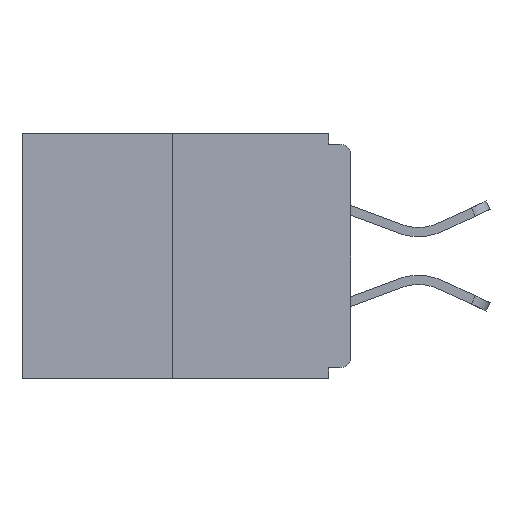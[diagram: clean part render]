
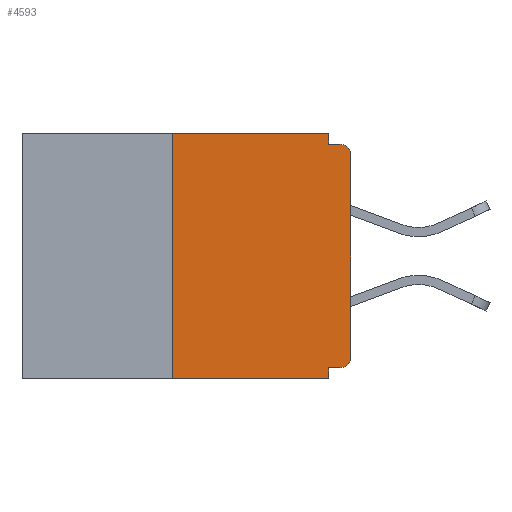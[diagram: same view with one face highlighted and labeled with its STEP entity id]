
A CAD part, left-side view. The second image highlights one B-rep face of the part: STEP entity #4593.
In plain terms, the highlighted planar face has unit normal (-1, 0, 0).
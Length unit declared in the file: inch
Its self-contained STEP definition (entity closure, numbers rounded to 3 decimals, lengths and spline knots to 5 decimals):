
#441 = LINE ( 'NONE', #9095, #3530 ) ;
#461 = VERTEX_POINT ( 'NONE', #24183 ) ;
#647 = DIRECTION ( 'NONE',  ( 0., -1., 0. ) ) ;
#723 = CARTESIAN_POINT ( 'NONE',  ( 0., 0.25, -0.343 ) ) ;
#873 = ORIENTED_EDGE ( 'NONE', *, *, #22723, .T. ) ;
#1362 = AXIS2_PLACEMENT_3D ( 'NONE', #7257, #23128, #17271 ) ;
#1671 = CARTESIAN_POINT ( 'NONE',  ( 0., 0.25, 0. ) ) ;
#1833 = CIRCLE ( 'NONE', #21956, 0.015 ) ;
#2338 = CARTESIAN_POINT ( 'NONE',  ( 0., 0.46, 0. ) ) ;
#2675 = EDGE_CURVE ( 'NONE', #16763, #24442, #19767, .T. ) ;
#3530 = VECTOR ( 'NONE', #11097, 39.37008 ) ;
#3988 = DIRECTION ( 'NONE',  ( 0., 0., 1. ) ) ;
#4593 = ADVANCED_FACE ( 'NONE', ( #5600 ), #15111, .F. ) ;
#4710 = DIRECTION ( 'NONE',  ( -1., 0., 0. ) ) ;
#4755 = VECTOR ( 'NONE', #13720, 39.37008 ) ;
#5445 = DIRECTION ( 'NONE',  ( 0., 0., -1. ) ) ;
#5600 = FACE_OUTER_BOUND ( 'NONE', #6929, .T. ) ;
#5951 = CARTESIAN_POINT ( 'NONE',  ( 0., 0., -0.015 ) ) ;
#6776 = CARTESIAN_POINT ( 'NONE',  ( 0., 0.031, -0.343 ) ) ;
#6848 = CARTESIAN_POINT ( 'NONE',  ( 0., 0.031, -0.343 ) ) ;
#6924 = CARTESIAN_POINT ( 'NONE',  ( 0., 0.031, 0. ) ) ;
#6929 = EDGE_LOOP ( 'NONE', ( #24272, #15865, #21165, #22996, #10280, #16289, #873, #14634, #24506, #10809 ) ) ;
#7257 = CARTESIAN_POINT ( 'NONE',  ( 0., 0.46, 0. ) ) ;
#7314 = CARTESIAN_POINT ( 'NONE',  ( 0., 0.015, -0.015 ) ) ;
#7361 = CARTESIAN_POINT ( 'NONE',  ( 0., 0.031, 0. ) ) ;
#7460 = LINE ( 'NONE', #6848, #10587 ) ;
#8065 = DIRECTION ( 'NONE',  ( 0., 0., -1. ) ) ;
#8109 = CARTESIAN_POINT ( 'NONE',  ( 0., 0., 0. ) ) ;
#8378 = DIRECTION ( 'NONE',  ( 0., -1., 0. ) ) ;
#8689 = VERTEX_POINT ( 'NONE', #7361 ) ;
#9004 = VECTOR ( 'NONE', #647, 39.37008 ) ;
#9095 = CARTESIAN_POINT ( 'NONE',  ( 0., 0.25, 0. ) ) ;
#9222 = EDGE_CURVE ( 'NONE', #15739, #12698, #18220, .T. ) ;
#9432 = VERTEX_POINT ( 'NONE', #9999 ) ;
#9542 = CARTESIAN_POINT ( 'NONE',  ( 0., 0.031, -0.328 ) ) ;
#9869 = CARTESIAN_POINT ( 'NONE',  ( 0., 0.031, -0.015 ) ) ;
#9999 = CARTESIAN_POINT ( 'NONE',  ( 0., 0., -0.03 ) ) ;
#10280 = ORIENTED_EDGE ( 'NONE', *, *, #9222, .F. ) ;
#10587 = VECTOR ( 'NONE', #5445, 39.37008 ) ;
#10809 = ORIENTED_EDGE ( 'NONE', *, *, #21538, .F. ) ;
#11043 = LINE ( 'NONE', #2338, #20100 ) ;
#11097 = DIRECTION ( 'NONE',  ( 0., 0., 1. ) ) ;
#11209 = VERTEX_POINT ( 'NONE', #1671 ) ;
#11656 = DIRECTION ( 'NONE',  ( 0., 1., 0. ) ) ;
#11887 = DIRECTION ( 'NONE',  ( -1., 0., 0. ) ) ;
#12581 = EDGE_CURVE ( 'NONE', #12698, #21178, #7460, .T. ) ;
#12598 = DIRECTION ( 'NONE',  ( 0., 0., -1. ) ) ;
#12698 = VERTEX_POINT ( 'NONE', #9542 ) ;
#12739 = EDGE_CURVE ( 'NONE', #15739, #461, #19937, .T. ) ;
#12963 = EDGE_CURVE ( 'NONE', #20572, #21178, #23593, .T. ) ;
#13240 = AXIS2_PLACEMENT_3D ( 'NONE', #15998, #11887, #8065 ) ;
#13720 = DIRECTION ( 'NONE',  ( 0., -1., 0. ) ) ;
#14511 = VECTOR ( 'NONE', #12598, 39.37008 ) ;
#14634 = ORIENTED_EDGE ( 'NONE', *, *, #16588, .T. ) ;
#15111 = PLANE ( 'NONE',  #1362 ) ;
#15739 = VERTEX_POINT ( 'NONE', #17661 ) ;
#15865 = ORIENTED_EDGE ( 'NONE', *, *, #20062, .F. ) ;
#15998 = CARTESIAN_POINT ( 'NONE',  ( 0., 0.015, -0.313 ) ) ;
#16289 = ORIENTED_EDGE ( 'NONE', *, *, #12739, .T. ) ;
#16450 = DIRECTION ( 'NONE',  ( 0., 0., -1. ) ) ;
#16588 = EDGE_CURVE ( 'NONE', #9432, #24442, #1833, .T. ) ;
#16763 = VERTEX_POINT ( 'NONE', #9869 ) ;
#17271 = DIRECTION ( 'NONE',  ( 0., 0., -1. ) ) ;
#17661 = CARTESIAN_POINT ( 'NONE',  ( 0., 0.015, -0.328 ) ) ;
#17862 = LINE ( 'NONE', #8109, #20333 ) ;
#18220 = LINE ( 'NONE', #25186, #19460 ) ;
#19460 = VECTOR ( 'NONE', #11656, 39.37008 ) ;
#19732 = EDGE_CURVE ( 'NONE', #11209, #8689, #11043, .T. ) ;
#19767 = LINE ( 'NONE', #5951, #4755 ) ;
#19796 = LINE ( 'NONE', #6924, #14511 ) ;
#19937 = CIRCLE ( 'NONE', #13240, 0.015 ) ;
#20062 = EDGE_CURVE ( 'NONE', #20572, #11209, #441, .T. ) ;
#20100 = VECTOR ( 'NONE', #8378, 39.37008 ) ;
#20333 = VECTOR ( 'NONE', #3988, 39.37008 ) ;
#20572 = VERTEX_POINT ( 'NONE', #723 ) ;
#20582 = CARTESIAN_POINT ( 'NONE',  ( 0., 0.015, -0.03 ) ) ;
#21165 = ORIENTED_EDGE ( 'NONE', *, *, #12963, .T. ) ;
#21178 = VERTEX_POINT ( 'NONE', #6776 ) ;
#21538 = EDGE_CURVE ( 'NONE', #8689, #16763, #19796, .T. ) ;
#21956 = AXIS2_PLACEMENT_3D ( 'NONE', #20582, #4710, #16450 ) ;
#22723 = EDGE_CURVE ( 'NONE', #461, #9432, #17862, .T. ) ;
#22784 = CARTESIAN_POINT ( 'NONE',  ( 0., 0.46, -0.343 ) ) ;
#22996 = ORIENTED_EDGE ( 'NONE', *, *, #12581, .F. ) ;
#23128 = DIRECTION ( 'NONE',  ( 1., 0., 0. ) ) ;
#23593 = LINE ( 'NONE', #22784, #9004 ) ;
#24183 = CARTESIAN_POINT ( 'NONE',  ( 0., 0., -0.313 ) ) ;
#24272 = ORIENTED_EDGE ( 'NONE', *, *, #19732, .F. ) ;
#24442 = VERTEX_POINT ( 'NONE', #7314 ) ;
#24506 = ORIENTED_EDGE ( 'NONE', *, *, #2675, .F. ) ;
#25186 = CARTESIAN_POINT ( 'NONE',  ( 0., 0., -0.328 ) ) ;
